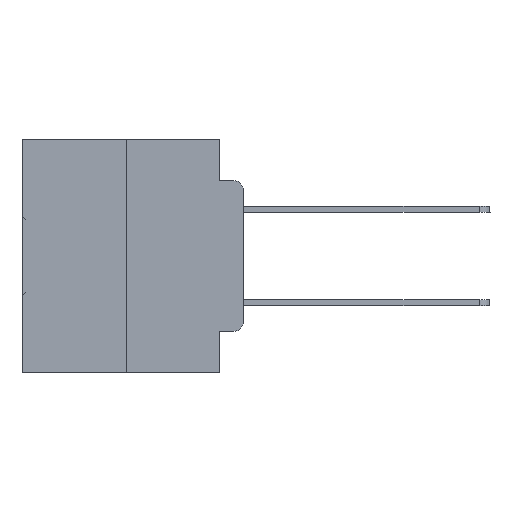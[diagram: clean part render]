
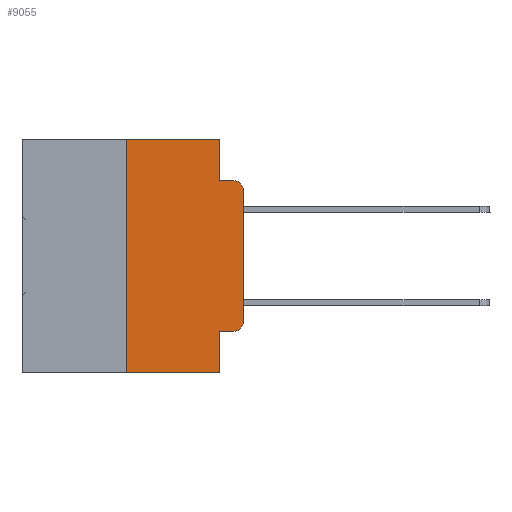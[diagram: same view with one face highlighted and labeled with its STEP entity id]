
A CAD part, left-side view. The second image highlights one B-rep face of the part: STEP entity #9055.
In plain terms, the highlighted planar face has unit normal (-1, 0, 0).
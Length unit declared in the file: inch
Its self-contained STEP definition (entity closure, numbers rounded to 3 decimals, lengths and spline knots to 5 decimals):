
#67 = CARTESIAN_POINT ( 'NONE',  ( 0., 0., -0.3915 ) ) ;
#544 = ORIENTED_EDGE ( 'NONE', *, *, #2865, .F. ) ;
#552 = VECTOR ( 'NONE', #33435, 39.37008 ) ;
#1017 = VERTEX_POINT ( 'NONE', #18928 ) ;
#1705 = LINE ( 'NONE', #12068, #33434 ) ;
#1992 = CARTESIAN_POINT ( 'NONE',  ( 0., 0.051, -0.4115 ) ) ;
#2161 = AXIS2_PLACEMENT_3D ( 'NONE', #10271, #7894, #20893 ) ;
#2814 = DIRECTION ( 'NONE',  ( 0., -1., 0. ) ) ;
#2865 = EDGE_CURVE ( 'NONE', #34276, #25762, #12627, .T. ) ;
#4416 = DIRECTION ( 'NONE',  ( 0., -1., 0. ) ) ;
#4609 = VERTEX_POINT ( 'NONE', #27517 ) ;
#4813 = VECTOR ( 'NONE', #16786, 39.37008 ) ;
#5297 = CARTESIAN_POINT ( 'NONE',  ( 0., 0.051, -0.4115 ) ) ;
#5437 = CARTESIAN_POINT ( 'NONE',  ( 0., 0.25, 0. ) ) ;
#5527 = VERTEX_POINT ( 'NONE', #14468 ) ;
#5672 = EDGE_CURVE ( 'NONE', #25762, #4609, #1705, .T. ) ;
#5765 = CARTESIAN_POINT ( 'NONE',  ( 0., 0.051, 0. ) ) ;
#6450 = CARTESIAN_POINT ( 'NONE',  ( 0., 0., -0.1085 ) ) ;
#7894 = DIRECTION ( 'NONE',  ( 1., 0., 0. ) ) ;
#8024 = VERTEX_POINT ( 'NONE', #11921 ) ;
#8053 = ORIENTED_EDGE ( 'NONE', *, *, #26867, .T. ) ;
#8547 = LINE ( 'NONE', #12104, #552 ) ;
#9055 = ADVANCED_FACE ( 'NONE', ( #26279 ), #23849, .F. ) ;
#10163 = ORIENTED_EDGE ( 'NONE', *, *, #26228, .T. ) ;
#10248 = LINE ( 'NONE', #31635, #21213 ) ;
#10271 = CARTESIAN_POINT ( 'NONE',  ( 0., 0.473, 0. ) ) ;
#10327 = CARTESIAN_POINT ( 'NONE',  ( 0., 0.02, -0.3915 ) ) ;
#11235 = ORIENTED_EDGE ( 'NONE', *, *, #19746, .T. ) ;
#11339 = DIRECTION ( 'NONE',  ( 0., 0., -1. ) ) ;
#11921 = CARTESIAN_POINT ( 'NONE',  ( 0., 0.051, -0.5 ) ) ;
#12068 = CARTESIAN_POINT ( 'NONE',  ( 0., 0.473, 0. ) ) ;
#12104 = CARTESIAN_POINT ( 'NONE',  ( 0., 0., 0. ) ) ;
#12202 = CARTESIAN_POINT ( 'NONE',  ( 0., 0.02, -0.4115 ) ) ;
#12627 = LINE ( 'NONE', #28015, #26164 ) ;
#12833 = LINE ( 'NONE', #5765, #32730 ) ;
#12890 = VECTOR ( 'NONE', #28947, 39.37008 ) ;
#13270 = VERTEX_POINT ( 'NONE', #12202 ) ;
#14468 = CARTESIAN_POINT ( 'NONE',  ( 0., 0.02, -0.0885 ) ) ;
#16098 = CARTESIAN_POINT ( 'NONE',  ( 0., 0.25, -0.5 ) ) ;
#16786 = DIRECTION ( 'NONE',  ( 0., 0., -1. ) ) ;
#17102 = ORIENTED_EDGE ( 'NONE', *, *, #21025, .F. ) ;
#17161 = AXIS2_PLACEMENT_3D ( 'NONE', #10327, #18473, #23660 ) ;
#18473 = DIRECTION ( 'NONE',  ( -1., 0., 0. ) ) ;
#18928 = CARTESIAN_POINT ( 'NONE',  ( 0., 0.051, -0.0885 ) ) ;
#19469 = ORIENTED_EDGE ( 'NONE', *, *, #21924, .F. ) ;
#19536 = AXIS2_PLACEMENT_3D ( 'NONE', #27617, #24990, #24637 ) ;
#19746 = EDGE_CURVE ( 'NONE', #13270, #19979, #23898, .T. ) ;
#19828 = CARTESIAN_POINT ( 'NONE',  ( 0., 0.051, 0. ) ) ;
#19979 = VERTEX_POINT ( 'NONE', #67 ) ;
#20170 = DIRECTION ( 'NONE',  ( 0., 0., 1. ) ) ;
#20893 = DIRECTION ( 'NONE',  ( 0., 0., -1. ) ) ;
#21025 = EDGE_CURVE ( 'NONE', #23859, #8024, #12833, .T. ) ;
#21213 = VECTOR ( 'NONE', #4416, 39.37008 ) ;
#21924 = EDGE_CURVE ( 'NONE', #1017, #5527, #10248, .T. ) ;
#23126 = ORIENTED_EDGE ( 'NONE', *, *, #32233, .T. ) ;
#23660 = DIRECTION ( 'NONE',  ( 0., 0., -1. ) ) ;
#23849 = PLANE ( 'NONE',  #2161 ) ;
#23859 = VERTEX_POINT ( 'NONE', #5297 ) ;
#23898 = CIRCLE ( 'NONE', #17161, 0.02 ) ;
#24637 = DIRECTION ( 'NONE',  ( 0., 0., -1. ) ) ;
#24684 = LINE ( 'NONE', #19828, #4813 ) ;
#24990 = DIRECTION ( 'NONE',  ( -1., 0., 0. ) ) ;
#25401 = DIRECTION ( 'NONE',  ( 0., -1., 0. ) ) ;
#25762 = VERTEX_POINT ( 'NONE', #5437 ) ;
#25835 = EDGE_CURVE ( 'NONE', #4609, #1017, #24684, .T. ) ;
#26164 = VECTOR ( 'NONE', #20170, 39.37008 ) ;
#26228 = EDGE_CURVE ( 'NONE', #34276, #8024, #27664, .T. ) ;
#26279 = FACE_OUTER_BOUND ( 'NONE', #29601, .T. ) ;
#26867 = EDGE_CURVE ( 'NONE', #19979, #29005, #8547, .T. ) ;
#27517 = CARTESIAN_POINT ( 'NONE',  ( 0., 0.051, 0. ) ) ;
#27617 = CARTESIAN_POINT ( 'NONE',  ( 0., 0.02, -0.1085 ) ) ;
#27664 = LINE ( 'NONE', #31807, #31068 ) ;
#28015 = CARTESIAN_POINT ( 'NONE',  ( 0., 0.25, 0. ) ) ;
#28947 = DIRECTION ( 'NONE',  ( 0., -1., 0. ) ) ;
#29005 = VERTEX_POINT ( 'NONE', #6450 ) ;
#29392 = LINE ( 'NONE', #1992, #12890 ) ;
#29601 = EDGE_LOOP ( 'NONE', ( #8053, #30490, #19469, #30300, #29661, #544, #10163, #17102, #23126, #11235 ) ) ;
#29661 = ORIENTED_EDGE ( 'NONE', *, *, #5672, .F. ) ;
#30300 = ORIENTED_EDGE ( 'NONE', *, *, #25835, .F. ) ;
#30490 = ORIENTED_EDGE ( 'NONE', *, *, #33694, .T. ) ;
#31068 = VECTOR ( 'NONE', #2814, 39.37008 ) ;
#31635 = CARTESIAN_POINT ( 'NONE',  ( 0., 0.051, -0.0885 ) ) ;
#31807 = CARTESIAN_POINT ( 'NONE',  ( 0., 0.473, -0.5 ) ) ;
#32233 = EDGE_CURVE ( 'NONE', #23859, #13270, #29392, .T. ) ;
#32730 = VECTOR ( 'NONE', #11339, 39.37008 ) ;
#33434 = VECTOR ( 'NONE', #25401, 39.37008 ) ;
#33435 = DIRECTION ( 'NONE',  ( 0., 0., 1. ) ) ;
#33694 = EDGE_CURVE ( 'NONE', #29005, #5527, #33941, .T. ) ;
#33941 = CIRCLE ( 'NONE', #19536, 0.02 ) ;
#34276 = VERTEX_POINT ( 'NONE', #16098 ) ;
